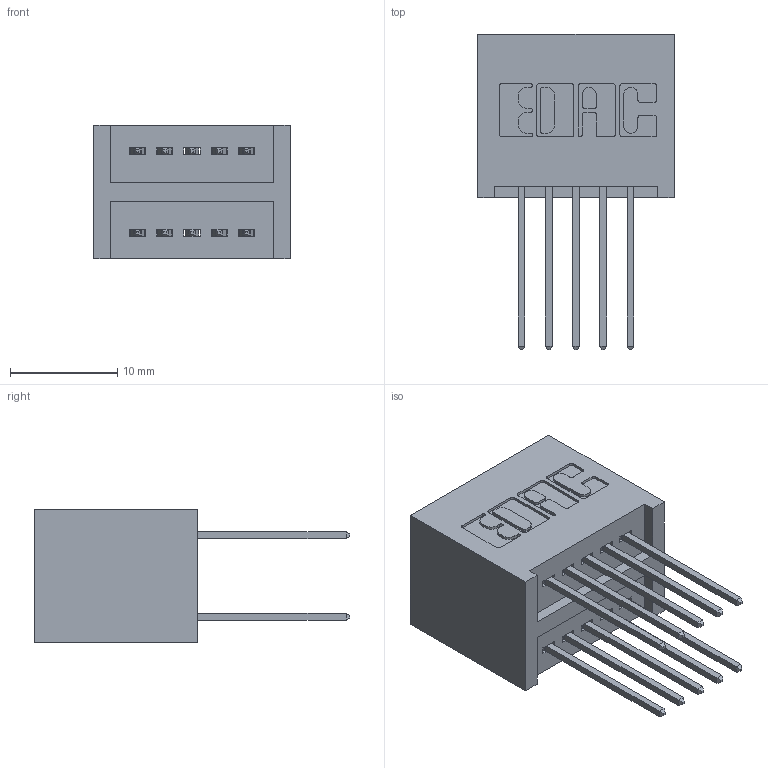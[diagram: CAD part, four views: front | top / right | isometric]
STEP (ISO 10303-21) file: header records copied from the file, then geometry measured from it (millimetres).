
FILE_DESCRIPTION (( 'STEP AP203' ), '1' );
FILE_NAME ('325-010-540-201.STEP', '2020-02-24T15:13:13', ( '' ), ( '' ), 'SwSTEP 2.0', 'SolidWorks 2016', '' );
FILE_SCHEMA (( 'CONFIG_CONTROL_DESIGN' ));
Length unit declared in the file: inch
Products named in the file (3): 325 Part_Lugless; 325-010-540-201; 325-292-001_325-293-140
Assembly tree (11 placements, depth 2):
  325-010-540-201
    325 Part_Lugless
    325-292-001_325-293-140  x10
Bounding box: 18.34 x 29.46 x 12.45 mm (x, y, z)
Volume: 2679.5 mm3; surface area: 3207.3 mm2
Topology: 11 solids, 11 shells, 626 faces, 1837 edges, 1210 vertices
Faces by surface type: plane 426, cylinder 200
Entity records: 7743 total; most frequent: CARTESIAN_POINT 1326, ORIENTED_EDGE 1262, DIRECTION 1191, EDGE_CURVE 631, VECTOR 511, LINE 511, VERTEX_POINT 418, AXIS2_PLACEMENT_3D 340
